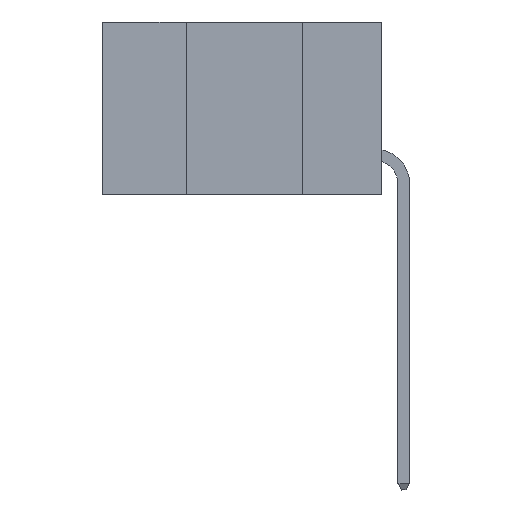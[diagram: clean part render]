
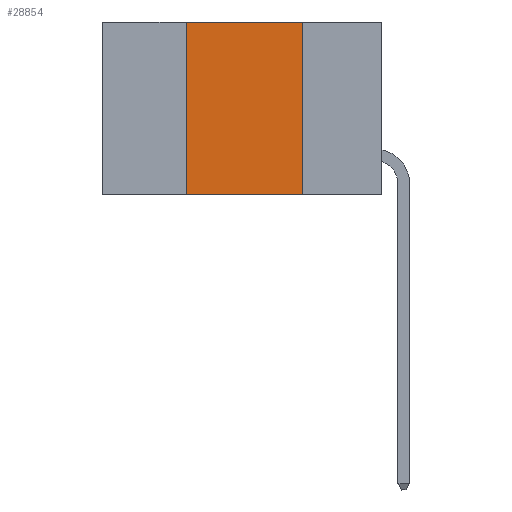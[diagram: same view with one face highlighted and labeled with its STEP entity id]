
A CAD part, left-side view. The second image highlights one B-rep face of the part: STEP entity #28854.
In plain terms, the highlighted planar face has unit normal (-1, 0, 0).
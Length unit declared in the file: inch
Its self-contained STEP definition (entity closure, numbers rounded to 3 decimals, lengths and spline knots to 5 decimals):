
#568 = VECTOR ( 'NONE', #3748, 39.37008 ) ;
#2308 = LINE ( 'NONE', #22785, #14615 ) ;
#3748 = DIRECTION ( 'NONE',  ( 0., 0., -1. ) ) ;
#5610 = VECTOR ( 'NONE', #29015, 39.37008 ) ;
#6197 = DIRECTION ( 'NONE',  ( 1., 0., 0. ) ) ;
#6974 = ORIENTED_EDGE ( 'NONE', *, *, #11906, .T. ) ;
#7125 = CARTESIAN_POINT ( 'NONE',  ( 0., 0.42, 0. ) ) ;
#7711 = VERTEX_POINT ( 'NONE', #7125 ) ;
#8598 = CARTESIAN_POINT ( 'NONE',  ( 0., 0.17, 0. ) ) ;
#8834 = ORIENTED_EDGE ( 'NONE', *, *, #11876, .F. ) ;
#9592 = CARTESIAN_POINT ( 'NONE',  ( 0., 0.17, 0. ) ) ;
#11876 = EDGE_CURVE ( 'NONE', #7711, #26526, #29724, .T. ) ;
#11906 = EDGE_CURVE ( 'NONE', #14344, #16397, #2308, .T. ) ;
#12927 = CARTESIAN_POINT ( 'NONE',  ( 0., 0.42, -0.37 ) ) ;
#13063 = CARTESIAN_POINT ( 'NONE',  ( 0., 0.6, 0. ) ) ;
#14344 = VERTEX_POINT ( 'NONE', #12927 ) ;
#14615 = VECTOR ( 'NONE', #32318, 39.37008 ) ;
#16397 = VERTEX_POINT ( 'NONE', #32199 ) ;
#16438 = VECTOR ( 'NONE', #38675, 39.37008 ) ;
#17530 = ORIENTED_EDGE ( 'NONE', *, *, #25417, .F. ) ;
#21027 = AXIS2_PLACEMENT_3D ( 'NONE', #24244, #6197, #27291 ) ;
#22785 = CARTESIAN_POINT ( 'NONE',  ( 0., 0.6, -0.37 ) ) ;
#23559 = FACE_OUTER_BOUND ( 'NONE', #35675, .T. ) ;
#24244 = CARTESIAN_POINT ( 'NONE',  ( 0., 0.6, 0. ) ) ;
#24639 = LINE ( 'NONE', #9592, #568 ) ;
#25417 = EDGE_CURVE ( 'NONE', #14344, #7711, #32491, .T. ) ;
#26526 = VERTEX_POINT ( 'NONE', #8598 ) ;
#27291 = DIRECTION ( 'NONE',  ( 0., 0., -1. ) ) ;
#27594 = ORIENTED_EDGE ( 'NONE', *, *, #32202, .F. ) ;
#28854 = ADVANCED_FACE ( 'NONE', ( #23559 ), #39130, .F. ) ;
#29015 = DIRECTION ( 'NONE',  ( 0., -1., 0. ) ) ;
#29724 = LINE ( 'NONE', #13063, #5610 ) ;
#32199 = CARTESIAN_POINT ( 'NONE',  ( 0., 0.17, -0.37 ) ) ;
#32202 = EDGE_CURVE ( 'NONE', #26526, #16397, #24639, .T. ) ;
#32318 = DIRECTION ( 'NONE',  ( 0., -1., 0. ) ) ;
#32491 = LINE ( 'NONE', #39198, #16438 ) ;
#35675 = EDGE_LOOP ( 'NONE', ( #27594, #8834, #17530, #6974 ) ) ;
#38675 = DIRECTION ( 'NONE',  ( 0., 0., 1. ) ) ;
#39130 = PLANE ( 'NONE',  #21027 ) ;
#39198 = CARTESIAN_POINT ( 'NONE',  ( 0., 0.42, 0. ) ) ;
